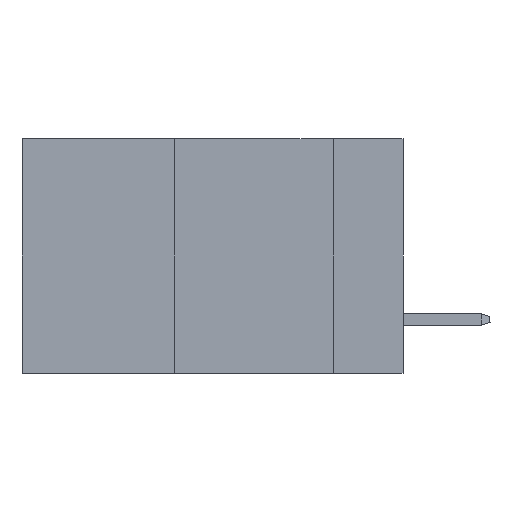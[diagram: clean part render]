
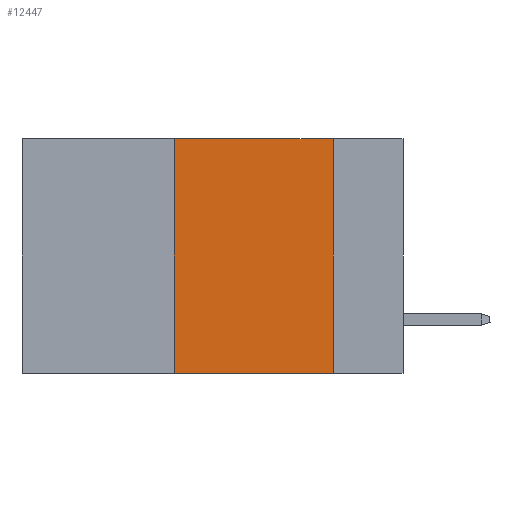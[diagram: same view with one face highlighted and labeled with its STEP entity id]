
A CAD part, left-side view. The second image highlights one B-rep face of the part: STEP entity #12447.
In plain terms, the highlighted planar face has unit normal (-1, 0, 0).
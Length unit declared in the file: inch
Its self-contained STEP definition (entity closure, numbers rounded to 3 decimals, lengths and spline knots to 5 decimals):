
#133 = CARTESIAN_POINT ( 'NONE',  ( 0., 0.36, 0. ) ) ;
#804 = ORIENTED_EDGE ( 'NONE', *, *, #20253, .F. ) ;
#1080 = DIRECTION ( 'NONE',  ( 0., -1., 0. ) ) ;
#1565 = VECTOR ( 'NONE', #5322, 39.37008 ) ;
#1912 = EDGE_LOOP ( 'NONE', ( #804, #17010, #16588, #16448 ) ) ;
#5057 = CARTESIAN_POINT ( 'NONE',  ( 0., 0.6, -0.37 ) ) ;
#5322 = DIRECTION ( 'NONE',  ( 0., 0., -1. ) ) ;
#5413 = CARTESIAN_POINT ( 'NONE',  ( 0., 0.36, -0.37 ) ) ;
#6506 = VECTOR ( 'NONE', #6687, 39.37008 ) ;
#6687 = DIRECTION ( 'NONE',  ( 0., -1., 0. ) ) ;
#7181 = LINE ( 'NONE', #12421, #1565 ) ;
#7893 = VERTEX_POINT ( 'NONE', #133 ) ;
#8339 = CARTESIAN_POINT ( 'NONE',  ( 0., 0.6, 0. ) ) ;
#8696 = AXIS2_PLACEMENT_3D ( 'NONE', #17104, #22498, #13357 ) ;
#11812 = PLANE ( 'NONE',  #8696 ) ;
#11993 = VECTOR ( 'NONE', #14920, 39.37008 ) ;
#12144 = LINE ( 'NONE', #5057, #6506 ) ;
#12421 = CARTESIAN_POINT ( 'NONE',  ( 0., 0.11, 0. ) ) ;
#12447 = ADVANCED_FACE ( 'NONE', ( #20523 ), #11812, .F. ) ;
#12482 = VECTOR ( 'NONE', #1080, 39.37008 ) ;
#13156 = LINE ( 'NONE', #20199, #11993 ) ;
#13357 = DIRECTION ( 'NONE',  ( 0., 0., -1. ) ) ;
#14750 = EDGE_CURVE ( 'NONE', #17250, #18738, #12144, .T. ) ;
#14920 = DIRECTION ( 'NONE',  ( 0., 0., 1. ) ) ;
#16112 = EDGE_CURVE ( 'NONE', #7893, #17223, #20875, .T. ) ;
#16313 = CARTESIAN_POINT ( 'NONE',  ( 0., 0.11, 0. ) ) ;
#16448 = ORIENTED_EDGE ( 'NONE', *, *, #14750, .T. ) ;
#16588 = ORIENTED_EDGE ( 'NONE', *, *, #21494, .F. ) ;
#16755 = CARTESIAN_POINT ( 'NONE',  ( 0., 0.11, -0.37 ) ) ;
#17010 = ORIENTED_EDGE ( 'NONE', *, *, #16112, .F. ) ;
#17104 = CARTESIAN_POINT ( 'NONE',  ( 0., 0.6, 0. ) ) ;
#17223 = VERTEX_POINT ( 'NONE', #16313 ) ;
#17250 = VERTEX_POINT ( 'NONE', #5413 ) ;
#18738 = VERTEX_POINT ( 'NONE', #16755 ) ;
#20199 = CARTESIAN_POINT ( 'NONE',  ( 0., 0.36, 0. ) ) ;
#20253 = EDGE_CURVE ( 'NONE', #17223, #18738, #7181, .T. ) ;
#20523 = FACE_OUTER_BOUND ( 'NONE', #1912, .T. ) ;
#20875 = LINE ( 'NONE', #8339, #12482 ) ;
#21494 = EDGE_CURVE ( 'NONE', #17250, #7893, #13156, .T. ) ;
#22498 = DIRECTION ( 'NONE',  ( 1., 0., 0. ) ) ;
